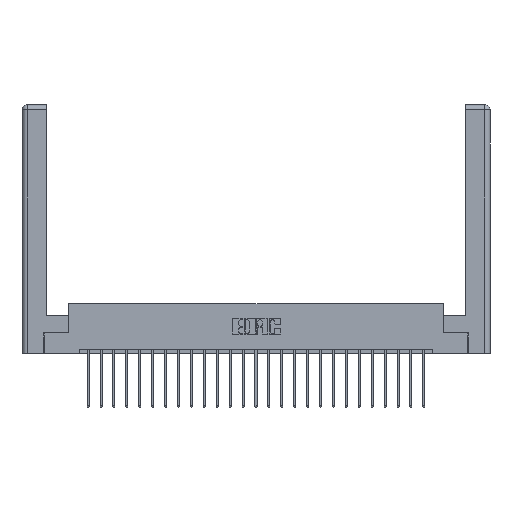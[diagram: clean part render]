
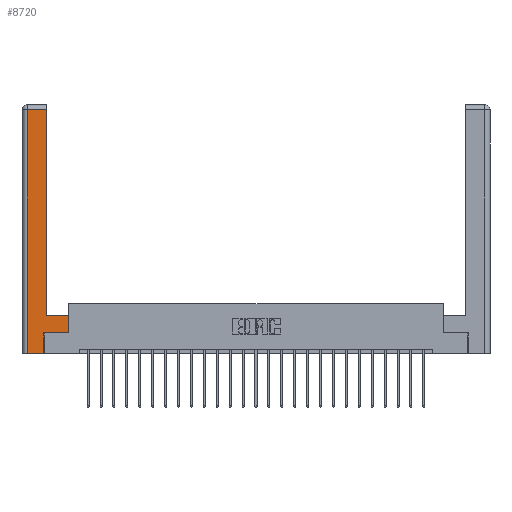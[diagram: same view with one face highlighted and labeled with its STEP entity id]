
A CAD part, top view. The second image highlights one B-rep face of the part: STEP entity #8720.
In plain terms, the highlighted planar face has unit normal (0, 0, 1).
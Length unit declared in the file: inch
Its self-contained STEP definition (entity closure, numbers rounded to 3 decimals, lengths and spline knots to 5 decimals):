
#355 = CARTESIAN_POINT ( 'NONE',  ( 0.0615, 2.94, 0. ) ) ;
#630 = DIRECTION ( 'NONE',  ( 1., 0., 0. ) ) ;
#805 = VECTOR ( 'NONE', #14274, 39.37008 ) ;
#983 = ORIENTED_EDGE ( 'NONE', *, *, #15440, .T. ) ;
#1425 = VERTEX_POINT ( 'NONE', #12954 ) ;
#1488 = EDGE_LOOP ( 'NONE', ( #16879, #22647, #19447, #5019, #983, #3614, #24241, #21878 ) ) ;
#1752 = LINE ( 'NONE', #18421, #805 ) ;
#2846 = LINE ( 'NONE', #13669, #18885 ) ;
#2887 = VECTOR ( 'NONE', #19668, 39.37008 ) ;
#3422 = EDGE_CURVE ( 'NONE', #24764, #1425, #2846, .T. ) ;
#3614 = ORIENTED_EDGE ( 'NONE', *, *, #21980, .T. ) ;
#3694 = PLANE ( 'NONE',  #8622 ) ;
#4199 = CARTESIAN_POINT ( 'NONE',  ( 0.265, 0.245, 0. ) ) ;
#4303 = CARTESIAN_POINT ( 'NONE',  ( 0.0615, 0., 0. ) ) ;
#5019 = ORIENTED_EDGE ( 'NONE', *, *, #6761, .T. ) ;
#5039 = VECTOR ( 'NONE', #630, 39.37008 ) ;
#5206 = LINE ( 'NONE', #9478, #13843 ) ;
#5413 = EDGE_CURVE ( 'NONE', #12729, #24909, #5828, .T. ) ;
#5828 = LINE ( 'NONE', #8032, #10451 ) ;
#5960 = DIRECTION ( 'NONE',  ( 0., 1., 0. ) ) ;
#6761 = EDGE_CURVE ( 'NONE', #25531, #15477, #13390, .T. ) ;
#7051 = VERTEX_POINT ( 'NONE', #15049 ) ;
#7332 = CARTESIAN_POINT ( 'NONE',  ( 0.265, 0., 0. ) ) ;
#7430 = DIRECTION ( 'NONE',  ( 0., 1., 0. ) ) ;
#8032 = CARTESIAN_POINT ( 'NONE',  ( 0.295, 3., 0. ) ) ;
#8622 = AXIS2_PLACEMENT_3D ( 'NONE', #21296, #19387, #9603 ) ;
#8720 = ADVANCED_FACE ( 'NONE', ( #12715 ), #3694, .F. ) ;
#9478 = CARTESIAN_POINT ( 'NONE',  ( 0.265, 0.245, 0. ) ) ;
#9603 = DIRECTION ( 'NONE',  ( -1., 0., 0. ) ) ;
#10215 = CARTESIAN_POINT ( 'NONE',  ( 0.265, 0., 0. ) ) ;
#10451 = VECTOR ( 'NONE', #5960, 39.37008 ) ;
#11267 = LINE ( 'NONE', #4303, #14655 ) ;
#12150 = CARTESIAN_POINT ( 'NONE',  ( 0.0615, 0., 0. ) ) ;
#12715 = FACE_OUTER_BOUND ( 'NONE', #1488, .T. ) ;
#12729 = VERTEX_POINT ( 'NONE', #13284 ) ;
#12954 = CARTESIAN_POINT ( 'NONE',  ( 0.565, 0.45, 0. ) ) ;
#12974 = EDGE_CURVE ( 'NONE', #7051, #25531, #11267, .T. ) ;
#13089 = LINE ( 'NONE', #21724, #2887 ) ;
#13284 = CARTESIAN_POINT ( 'NONE',  ( 0.295, 0.45, 0. ) ) ;
#13390 = LINE ( 'NONE', #10215, #5039 ) ;
#13669 = CARTESIAN_POINT ( 'NONE',  ( 0.565, 0.45, 0. ) ) ;
#13843 = VECTOR ( 'NONE', #7430, 39.37008 ) ;
#14169 = DIRECTION ( 'NONE',  ( -1., 0., 0. ) ) ;
#14274 = DIRECTION ( 'NONE',  ( 1., 0., 0. ) ) ;
#14655 = VECTOR ( 'NONE', #21995, 39.37008 ) ;
#15049 = CARTESIAN_POINT ( 'NONE',  ( 0.0615, 2.94, 0. ) ) ;
#15440 = EDGE_CURVE ( 'NONE', #15477, #16367, #5206, .T. ) ;
#15477 = VERTEX_POINT ( 'NONE', #7332 ) ;
#16298 = CARTESIAN_POINT ( 'NONE',  ( 0.295, 2.94, 0. ) ) ;
#16367 = VERTEX_POINT ( 'NONE', #4199 ) ;
#16879 = ORIENTED_EDGE ( 'NONE', *, *, #5413, .T. ) ;
#18421 = CARTESIAN_POINT ( 'NONE',  ( 0.565, 0.245, 0. ) ) ;
#18885 = VECTOR ( 'NONE', #23823, 39.37008 ) ;
#19387 = DIRECTION ( 'NONE',  ( 0., 0., -1. ) ) ;
#19447 = ORIENTED_EDGE ( 'NONE', *, *, #12974, .T. ) ;
#19574 = VECTOR ( 'NONE', #14169, 39.37008 ) ;
#19668 = DIRECTION ( 'NONE',  ( -1., 0., 0. ) ) ;
#21296 = CARTESIAN_POINT ( 'NONE',  ( 0., 0., 0. ) ) ;
#21418 = CARTESIAN_POINT ( 'NONE',  ( 0.565, 0.245, 0. ) ) ;
#21724 = CARTESIAN_POINT ( 'NONE',  ( 0.295, 0.45, 0. ) ) ;
#21878 = ORIENTED_EDGE ( 'NONE', *, *, #23838, .T. ) ;
#21980 = EDGE_CURVE ( 'NONE', #16367, #24764, #1752, .T. ) ;
#21995 = DIRECTION ( 'NONE',  ( 0., -1., 0. ) ) ;
#22647 = ORIENTED_EDGE ( 'NONE', *, *, #24372, .T. ) ;
#23823 = DIRECTION ( 'NONE',  ( 0., 1., 0. ) ) ;
#23838 = EDGE_CURVE ( 'NONE', #1425, #12729, #13089, .T. ) ;
#24241 = ORIENTED_EDGE ( 'NONE', *, *, #3422, .T. ) ;
#24372 = EDGE_CURVE ( 'NONE', #24909, #7051, #24785, .T. ) ;
#24764 = VERTEX_POINT ( 'NONE', #21418 ) ;
#24785 = LINE ( 'NONE', #355, #19574 ) ;
#24909 = VERTEX_POINT ( 'NONE', #16298 ) ;
#25531 = VERTEX_POINT ( 'NONE', #12150 ) ;
